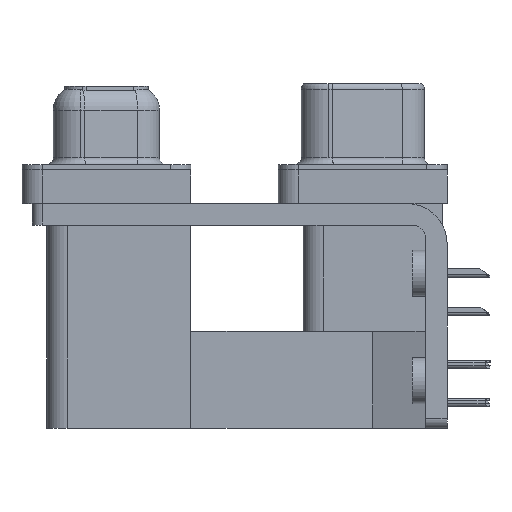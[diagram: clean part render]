
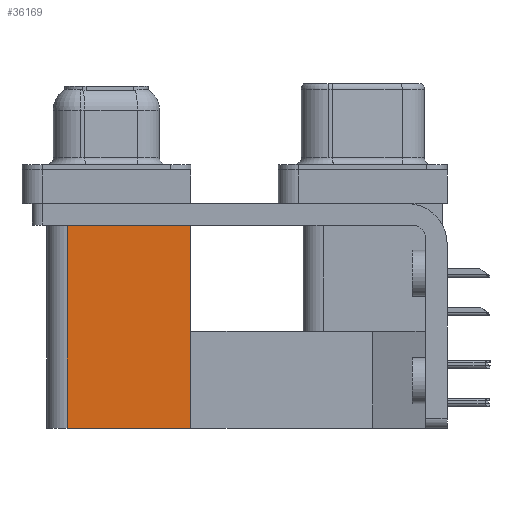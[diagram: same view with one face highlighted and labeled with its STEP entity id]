
A CAD part, left-side view. The second image highlights one B-rep face of the part: STEP entity #36169.
In plain terms, the highlighted planar face has unit normal (-1, 0, 0).
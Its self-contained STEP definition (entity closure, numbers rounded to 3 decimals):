
#96 = VECTOR ( 'NONE', #14544, 1000. ) ;
#640 = LINE ( 'NONE', #15541, #24384 ) ;
#2817 = CARTESIAN_POINT ( 'NONE',  ( 3.79, 12.775, -19.2 ) ) ;
#4464 = LINE ( 'NONE', #13750, #18051 ) ;
#4924 = EDGE_LOOP ( 'NONE', ( #13792, #19252, #26589, #32198 ) ) ;
#5816 = PLANE ( 'NONE',  #34658 ) ;
#6892 = EDGE_CURVE ( 'NONE', #10740, #14263, #4464, .T. ) ;
#6993 = EDGE_CURVE ( 'NONE', #10255, #10740, #39250, .T. ) ;
#8280 = VECTOR ( 'NONE', #8489, 1000. ) ;
#8489 = DIRECTION ( 'NONE',  ( 0., 0., 1. ) ) ;
#10012 = VERTEX_POINT ( 'NONE', #23352 ) ;
#10255 = VERTEX_POINT ( 'NONE', #24538 ) ;
#10740 = VERTEX_POINT ( 'NONE', #32309 ) ;
#11723 = CARTESIAN_POINT ( 'NONE',  ( 3.79, 12.775, -19.2 ) ) ;
#11880 = DIRECTION ( 'NONE',  ( 1., 0., 0. ) ) ;
#13119 = DIRECTION ( 'NONE',  ( 0., 1., 0. ) ) ;
#13750 = CARTESIAN_POINT ( 'NONE',  ( 3.79, 12.775, -2.5 ) ) ;
#13792 = ORIENTED_EDGE ( 'NONE', *, *, #6892, .T. ) ;
#14263 = VERTEX_POINT ( 'NONE', #31889 ) ;
#14544 = DIRECTION ( 'NONE',  ( 0., 0., 1. ) ) ;
#15541 = CARTESIAN_POINT ( 'NONE',  ( 3.79, 12.775, -19.2 ) ) ;
#18051 = VECTOR ( 'NONE', #34859, 1000. ) ;
#19060 = EDGE_CURVE ( 'NONE', #10255, #10012, #640, .T. ) ;
#19252 = ORIENTED_EDGE ( 'NONE', *, *, #35032, .F. ) ;
#23352 = CARTESIAN_POINT ( 'NONE',  ( 3.79, 21.975, -19.2 ) ) ;
#23920 = DIRECTION ( 'NONE',  ( 0., 1., 0. ) ) ;
#24358 = CARTESIAN_POINT ( 'NONE',  ( 3.79, 21.975, -19.2 ) ) ;
#24384 = VECTOR ( 'NONE', #13119, 1000. ) ;
#24538 = CARTESIAN_POINT ( 'NONE',  ( 3.79, 12.775, -19.2 ) ) ;
#26589 = ORIENTED_EDGE ( 'NONE', *, *, #19060, .F. ) ;
#27143 = FACE_OUTER_BOUND ( 'NONE', #4924, .T. ) ;
#31889 = CARTESIAN_POINT ( 'NONE',  ( 3.79, 21.975, -2.5 ) ) ;
#32198 = ORIENTED_EDGE ( 'NONE', *, *, #6993, .T. ) ;
#32309 = CARTESIAN_POINT ( 'NONE',  ( 3.79, 12.775, -2.5 ) ) ;
#34658 = AXIS2_PLACEMENT_3D ( 'NONE', #2817, #11880, #23920 ) ;
#34859 = DIRECTION ( 'NONE',  ( 0., 1., 0. ) ) ;
#35032 = EDGE_CURVE ( 'NONE', #10012, #14263, #38648, .T. ) ;
#36169 = ADVANCED_FACE ( 'NONE', ( #27143 ), #5816, .F. ) ;
#38648 = LINE ( 'NONE', #24358, #8280 ) ;
#39250 = LINE ( 'NONE', #11723, #96 ) ;
